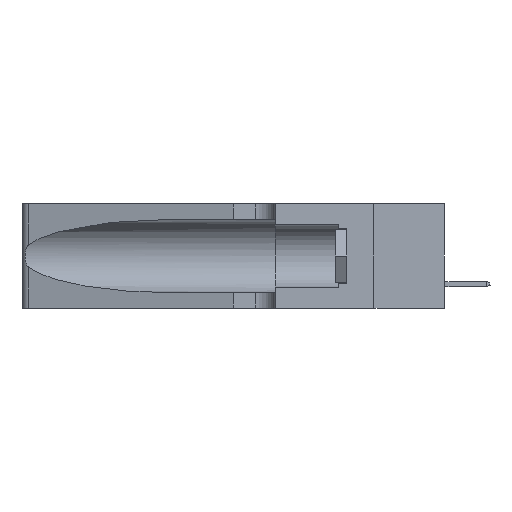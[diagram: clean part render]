
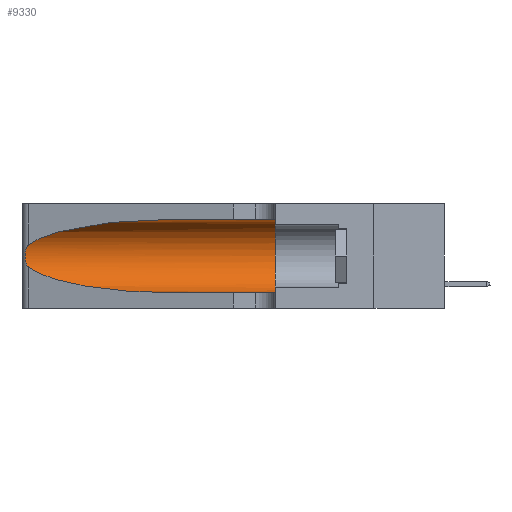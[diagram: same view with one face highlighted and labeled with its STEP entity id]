
A CAD part, left-side view. The second image highlights one B-rep face of the part: STEP entity #9330.
In plain terms, the highlighted cylindrical face has radius 3.308 mm (diameter 6.617 mm), a partial arc.
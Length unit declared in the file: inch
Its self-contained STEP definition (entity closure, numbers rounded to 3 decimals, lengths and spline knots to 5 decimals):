
#154 = CARTESIAN_POINT ( 'NONE',  ( 0.25639, 1.23184, 0.21858 ) ) ;
#2152 = CARTESIAN_POINT ( 'NONE',  ( 0.25639, 1.23186, 0.15144 ) ) ;
#2155 = FACE_OUTER_BOUND ( 'NONE', #4300, .T. ) ;
#2176 = ORIENTED_EDGE ( 'NONE', *, *, #7088, .F. ) ;
#2197 = VERTEX_POINT ( 'NONE', #16579 ) ;
#2857 = CARTESIAN_POINT ( 'NONE',  ( 0.25487, 1.22718, 0.22369 ) ) ;
#3127 = CARTESIAN_POINT ( 'NONE',  ( 0.18966, 0.96281, 0.05475 ) ) ;
#3153 = ORIENTED_EDGE ( 'NONE', *, *, #6195, .T. ) ;
#3188 = CARTESIAN_POINT ( 'NONE',  ( 0.25854, 1.2359, 0.20912 ) ) ;
#3243 = LINE ( 'NONE', #3245, #18876 ) ;
#3245 = CARTESIAN_POINT ( 'NONE',  ( 0.1305, 1.61858, 0.31525 ) ) ;
#3323 = CIRCLE ( 'NONE', #9309, 0.13025 ) ;
#3472 = DIRECTION ( 'NONE',  ( 0., -1., 0. ) ) ;
#4300 = EDGE_LOOP ( 'NONE', ( #11876, #11969, #15759, #3153, #11771, #2176 ) ) ;
#4462 = EDGE_CURVE ( 'NONE', #10695, #9946, #20226, .T. ) ;
#4940 = CARTESIAN_POINT ( 'NONE',  ( 0.25787, 1.23484, 0.2124 ) ) ;
#6195 = EDGE_CURVE ( 'NONE', #6870, #2197, #13300, .T. ) ;
#6391 = CARTESIAN_POINT ( 'NONE',  ( 0.26075, 1.23896, 0.178 ) ) ;
#6641 = DIRECTION ( 'NONE',  ( 0., 0., -1. ) ) ;
#6870 = VERTEX_POINT ( 'NONE', #15767 ) ;
#7088 = EDGE_CURVE ( 'NONE', #10695, #18698, #3243, .T. ) ;
#9309 = AXIS2_PLACEMENT_3D ( 'NONE', #14514, #16082, #10237 ) ;
#9330 = ADVANCED_FACE ( 'NONE', ( #2155 ), #19272, .F. ) ;
#9334 = CARTESIAN_POINT ( 'NONE',  ( 0.1305, 0.35, 0.31525 ) ) ;
#9456 = CARTESIAN_POINT ( 'NONE',  ( 0.25487, 1.22718, 0.22369 ) ) ;
#9502 = CARTESIAN_POINT ( 'NONE',  ( 0.1305, 0.72297, 0.05475 ) ) ;
#9946 = VERTEX_POINT ( 'NONE', #9456 ) ;
#10237 = DIRECTION ( 'NONE',  ( 0., 0., 1. ) ) ;
#10695 = VERTEX_POINT ( 'NONE', #17955 ) ;
#10735 = EDGE_CURVE ( 'NONE', #17849, #6870, #19608, .T. ) ;
#10900 = VECTOR ( 'NONE', #14006, 39.37008 ) ;
#11135 = CARTESIAN_POINT ( 'NONE',  ( 0.1305, 1.61858, 0.185 ) ) ;
#11358 = EDGE_CURVE ( 'NONE', #9946, #17849, #14251, .T. ) ;
#11771 = ORIENTED_EDGE ( 'NONE', *, *, #14873, .F. ) ;
#11876 = ORIENTED_EDGE ( 'NONE', *, *, #4462, .T. ) ;
#11969 = ORIENTED_EDGE ( 'NONE', *, *, #11358, .T. ) ;
#12772 = CARTESIAN_POINT ( 'NONE',  ( 0.1305, 0.72297, 0.31525 ) ) ;
#12831 = CARTESIAN_POINT ( 'NONE',  ( 0.2373, 1.15595, 0.28018 ) ) ;
#13034 = CARTESIAN_POINT ( 'NONE',  ( 0.25555, 1.22993, 0.14849 ) ) ;
#13300 = LINE ( 'NONE', #15637, #10900 ) ;
#13408 = CARTESIAN_POINT ( 'NONE',  ( 0.2373, 1.15595, 0.08982 ) ) ;
#14006 = DIRECTION ( 'NONE',  ( 0., -1., 0. ) ) ;
#14251 = B_SPLINE_CURVE_WITH_KNOTS ( 'NONE', 3,
 ( #2857, #14338, #154, #4940, #3188, #17443, #19034, #6391, #17580, #17779, #16099, #2152, #13034, #19441 ),
 .UNSPECIFIED., .F., .F.,
 ( 4, 2, 2, 2, 2, 2, 4 ),
 ( 0., 0.00027, 0.00053, 0.00107, 0.0016, 0.00187, 0.00214 ),
 .UNSPECIFIED. ) ;
#14338 = CARTESIAN_POINT ( 'NONE',  ( 0.25555, 1.22994, 0.2215 ) ) ;
#14514 = CARTESIAN_POINT ( 'NONE',  ( 0.1305, 0.35, 0.185 ) ) ;
#14873 = EDGE_CURVE ( 'NONE', #18698, #2197, #3323, .T. ) ;
#15637 = CARTESIAN_POINT ( 'NONE',  ( 0.1305, 1.61858, 0.05475 ) ) ;
#15759 = ORIENTED_EDGE ( 'NONE', *, *, #10735, .T. ) ;
#15765 = CARTESIAN_POINT ( 'NONE',  ( 0.25487, 1.22718, 0.14631 ) ) ;
#15767 = CARTESIAN_POINT ( 'NONE',  ( 0.1305, 0.72297, 0.05475 ) ) ;
#15977 = CARTESIAN_POINT ( 'NONE',  ( 0.18966, 0.96281, 0.31525 ) ) ;
#16082 = DIRECTION ( 'NONE',  ( 0., 1., 0. ) ) ;
#16099 = CARTESIAN_POINT ( 'NONE',  ( 0.25789, 1.23486, 0.15765 ) ) ;
#16579 = CARTESIAN_POINT ( 'NONE',  ( 0.1305, 0.35, 0.05475 ) ) ;
#17443 = CARTESIAN_POINT ( 'NONE',  ( 0.26018, 1.23835, 0.19895 ) ) ;
#17580 = CARTESIAN_POINT ( 'NONE',  ( 0.26017, 1.23833, 0.17102 ) ) ;
#17779 = CARTESIAN_POINT ( 'NONE',  ( 0.25856, 1.23593, 0.16098 ) ) ;
#17849 = VERTEX_POINT ( 'NONE', #15765 ) ;
#17955 = CARTESIAN_POINT ( 'NONE',  ( 0.1305, 0.72297, 0.31525 ) ) ;
#18029 = AXIS2_PLACEMENT_3D ( 'NONE', #11135, #3472, #6641 ) ;
#18698 = VERTEX_POINT ( 'NONE', #9334 ) ;
#18876 = VECTOR ( 'NONE', #18947, 39.37008 ) ;
#18892 = CARTESIAN_POINT ( 'NONE',  ( 0.25487, 1.22718, 0.22369 ) ) ;
#18947 = DIRECTION ( 'NONE',  ( 0., -1., 0. ) ) ;
#19034 = CARTESIAN_POINT ( 'NONE',  ( 0.26075, 1.23896, 0.19203 ) ) ;
#19272 = CYLINDRICAL_SURFACE ( 'NONE', #18029, 0.13025 ) ;
#19441 = CARTESIAN_POINT ( 'NONE',  ( 0.25487, 1.22718, 0.14631 ) ) ;
#19608 =( BOUNDED_CURVE ( )  B_SPLINE_CURVE ( 3, ( #19746, #13408, #3127, #9502 ),
 .UNSPECIFIED., .F., .F. ) 
 B_SPLINE_CURVE_WITH_KNOTS ( ( 4, 4 ),
 ( 3.44316, 4.71239 ),
 .UNSPECIFIED. ) 
 CURVE ( )  GEOMETRIC_REPRESENTATION_ITEM ( )  RATIONAL_B_SPLINE_CURVE ( ( 1., 0.87, 0.87, 1. ) ) 
 REPRESENTATION_ITEM ( '' )  );
#19746 = CARTESIAN_POINT ( 'NONE',  ( 0.25487, 1.22718, 0.14631 ) ) ;
#20226 =( BOUNDED_CURVE ( )  B_SPLINE_CURVE ( 3, ( #12772, #15977, #12831, #18892 ),
 .UNSPECIFIED., .F., .F. ) 
 B_SPLINE_CURVE_WITH_KNOTS ( ( 4, 4 ),
 ( 1.5708, 2.84003 ),
 .UNSPECIFIED. ) 
 CURVE ( )  GEOMETRIC_REPRESENTATION_ITEM ( )  RATIONAL_B_SPLINE_CURVE ( ( 1., 0.87, 0.87, 1. ) ) 
 REPRESENTATION_ITEM ( '' )  );
